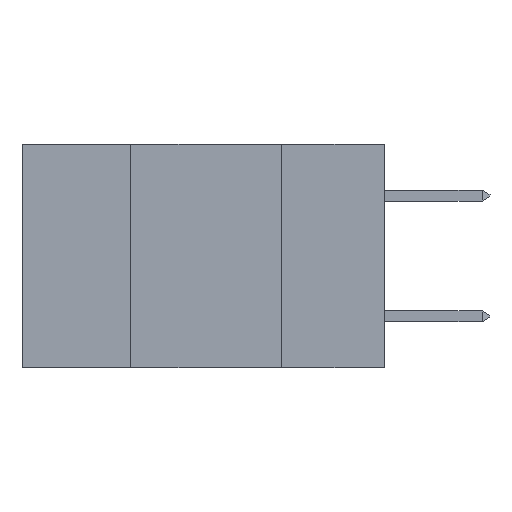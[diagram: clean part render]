
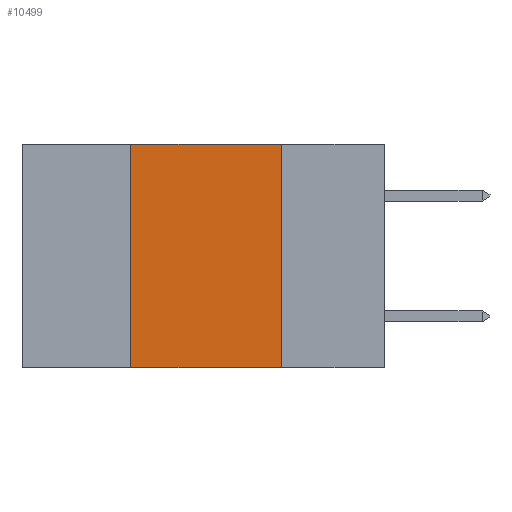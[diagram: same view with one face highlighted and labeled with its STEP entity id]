
A CAD part, left-side view. The second image highlights one B-rep face of the part: STEP entity #10499.
In plain terms, the highlighted planar face has unit normal (-1, 0, 0).
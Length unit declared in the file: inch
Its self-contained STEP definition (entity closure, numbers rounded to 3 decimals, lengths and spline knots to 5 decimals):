
#700 = VECTOR ( 'NONE', #1231, 39.37008 ) ;
#809 = ORIENTED_EDGE ( 'NONE', *, *, #1787, .F. ) ;
#1051 = VERTEX_POINT ( 'NONE', #2337 ) ;
#1191 = ORIENTED_EDGE ( 'NONE', *, *, #9895, .F. ) ;
#1231 = DIRECTION ( 'NONE',  ( 0., 0., -1. ) ) ;
#1787 = EDGE_CURVE ( 'NONE', #11475, #1051, #8088, .T. ) ;
#2337 = CARTESIAN_POINT ( 'NONE',  ( 0., 0.17, -0.37 ) ) ;
#3103 = CARTESIAN_POINT ( 'NONE',  ( 0., 0.42, 0. ) ) ;
#3279 = CARTESIAN_POINT ( 'NONE',  ( 0., 0.42, -0.37 ) ) ;
#4168 = PLANE ( 'NONE',  #12020 ) ;
#4505 = DIRECTION ( 'NONE',  ( 0., 0., 1. ) ) ;
#4693 = VERTEX_POINT ( 'NONE', #3103 ) ;
#4735 = CARTESIAN_POINT ( 'NONE',  ( 0., 0.6, 0. ) ) ;
#4914 = VECTOR ( 'NONE', #9863, 39.37008 ) ;
#4935 = LINE ( 'NONE', #4735, #7294 ) ;
#5388 = DIRECTION ( 'NONE',  ( 1., 0., 0. ) ) ;
#5775 = VERTEX_POINT ( 'NONE', #3279 ) ;
#6250 = LINE ( 'NONE', #9266, #11628 ) ;
#6616 = ORIENTED_EDGE ( 'NONE', *, *, #12580, .F. ) ;
#7294 = VECTOR ( 'NONE', #12793, 39.37008 ) ;
#7829 = DIRECTION ( 'NONE',  ( 0., 0., -1. ) ) ;
#8088 = LINE ( 'NONE', #13863, #700 ) ;
#8687 = ORIENTED_EDGE ( 'NONE', *, *, #12849, .T. ) ;
#9266 = CARTESIAN_POINT ( 'NONE',  ( 0., 0.42, 0. ) ) ;
#9863 = DIRECTION ( 'NONE',  ( 0., -1., 0. ) ) ;
#9895 = EDGE_CURVE ( 'NONE', #5775, #4693, #6250, .T. ) ;
#10103 = EDGE_LOOP ( 'NONE', ( #809, #6616, #1191, #8687 ) ) ;
#10499 = ADVANCED_FACE ( 'NONE', ( #12931 ), #4168, .F. ) ;
#11475 = VERTEX_POINT ( 'NONE', #12163 ) ;
#11628 = VECTOR ( 'NONE', #4505, 39.37008 ) ;
#12020 = AXIS2_PLACEMENT_3D ( 'NONE', #12221, #5388, #7829 ) ;
#12163 = CARTESIAN_POINT ( 'NONE',  ( 0., 0.17, 0. ) ) ;
#12221 = CARTESIAN_POINT ( 'NONE',  ( 0., 0.6, 0. ) ) ;
#12580 = EDGE_CURVE ( 'NONE', #4693, #11475, #4935, .T. ) ;
#12793 = DIRECTION ( 'NONE',  ( 0., -1., 0. ) ) ;
#12849 = EDGE_CURVE ( 'NONE', #5775, #1051, #12856, .T. ) ;
#12856 = LINE ( 'NONE', #14547, #4914 ) ;
#12931 = FACE_OUTER_BOUND ( 'NONE', #10103, .T. ) ;
#13863 = CARTESIAN_POINT ( 'NONE',  ( 0., 0.17, 0. ) ) ;
#14547 = CARTESIAN_POINT ( 'NONE',  ( 0., 0.6, -0.37 ) ) ;
